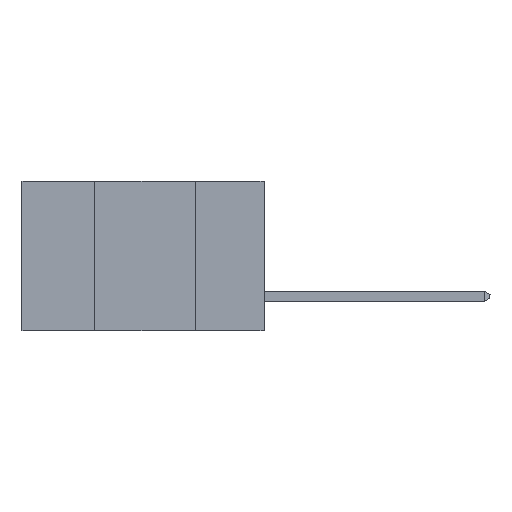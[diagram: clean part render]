
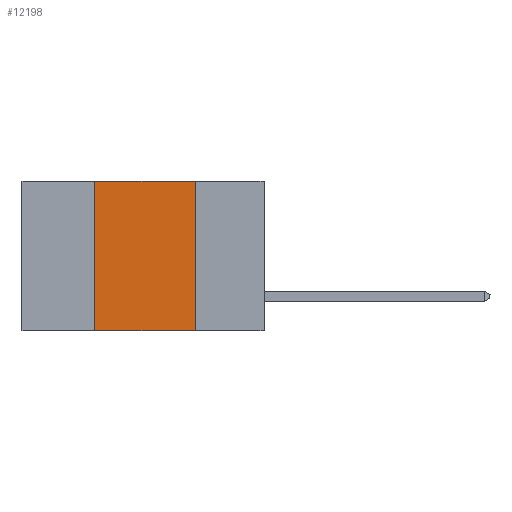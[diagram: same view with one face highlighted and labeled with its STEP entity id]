
A CAD part, left-side view. The second image highlights one B-rep face of the part: STEP entity #12198.
In plain terms, the highlighted planar face has unit normal (-1, 0, 0).
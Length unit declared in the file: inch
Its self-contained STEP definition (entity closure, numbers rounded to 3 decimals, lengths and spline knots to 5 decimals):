
#12 = DIRECTION ( 'NONE',  ( 1., 0., 0. ) ) ;
#21 = DIRECTION ( 'NONE',  ( 0., -1., 0. ) ) ;
#300 = FACE_OUTER_BOUND ( 'NONE', #9161, .T. ) ;
#1102 = EDGE_CURVE ( 'NONE', #4613, #13233, #21669, .T. ) ;
#1909 = VECTOR ( 'NONE', #21, 39.37008 ) ;
#3458 = DIRECTION ( 'NONE',  ( 0., -1., 0. ) ) ;
#3594 = DIRECTION ( 'NONE',  ( 0., 0., -1. ) ) ;
#4613 = VERTEX_POINT ( 'NONE', #22930 ) ;
#7232 = VECTOR ( 'NONE', #3594, 39.37008 ) ;
#7460 = CARTESIAN_POINT ( 'NONE',  ( 0., 0.17, -0.37 ) ) ;
#7839 = VECTOR ( 'NONE', #3458, 39.37008 ) ;
#9161 = EDGE_LOOP ( 'NONE', ( #11248, #14283, #9232, #23936 ) ) ;
#9232 = ORIENTED_EDGE ( 'NONE', *, *, #1102, .F. ) ;
#9684 = PLANE ( 'NONE',  #20125 ) ;
#10332 = CARTESIAN_POINT ( 'NONE',  ( 0., 0.42, 0. ) ) ;
#11082 = VECTOR ( 'NONE', #18038, 39.37008 ) ;
#11248 = ORIENTED_EDGE ( 'NONE', *, *, #19495, .F. ) ;
#12161 = LINE ( 'NONE', #13522, #1909 ) ;
#12198 = ADVANCED_FACE ( 'NONE', ( #300 ), #9684, .F. ) ;
#13233 = VERTEX_POINT ( 'NONE', #10332 ) ;
#13510 = DIRECTION ( 'NONE',  ( 0., 0., -1. ) ) ;
#13522 = CARTESIAN_POINT ( 'NONE',  ( 0., 0.6, 0. ) ) ;
#14283 = ORIENTED_EDGE ( 'NONE', *, *, #21979, .F. ) ;
#14848 = CARTESIAN_POINT ( 'NONE',  ( 0., 0.42, -0.37 ) ) ;
#14918 = CARTESIAN_POINT ( 'NONE',  ( 0., 0.6, -0.37 ) ) ;
#18038 = DIRECTION ( 'NONE',  ( 0., 0., 1. ) ) ;
#19495 = EDGE_CURVE ( 'NONE', #21838, #21106, #22364, .T. ) ;
#19775 = CARTESIAN_POINT ( 'NONE',  ( 0., 0.17, -0.37 ) ) ;
#20125 = AXIS2_PLACEMENT_3D ( 'NONE', #22877, #12, #13510 ) ;
#21106 = VERTEX_POINT ( 'NONE', #19775 ) ;
#21669 = LINE ( 'NONE', #14848, #11082 ) ;
#21838 = VERTEX_POINT ( 'NONE', #22219 ) ;
#21979 = EDGE_CURVE ( 'NONE', #13233, #21838, #12161, .T. ) ;
#22219 = CARTESIAN_POINT ( 'NONE',  ( 0., 0.17, 0. ) ) ;
#22345 = LINE ( 'NONE', #14918, #7839 ) ;
#22364 = LINE ( 'NONE', #7460, #7232 ) ;
#22877 = CARTESIAN_POINT ( 'NONE',  ( 0., 0.6, 0. ) ) ;
#22930 = CARTESIAN_POINT ( 'NONE',  ( 0., 0.42, -0.37 ) ) ;
#23813 = EDGE_CURVE ( 'NONE', #4613, #21106, #22345, .T. ) ;
#23936 = ORIENTED_EDGE ( 'NONE', *, *, #23813, .T. ) ;
